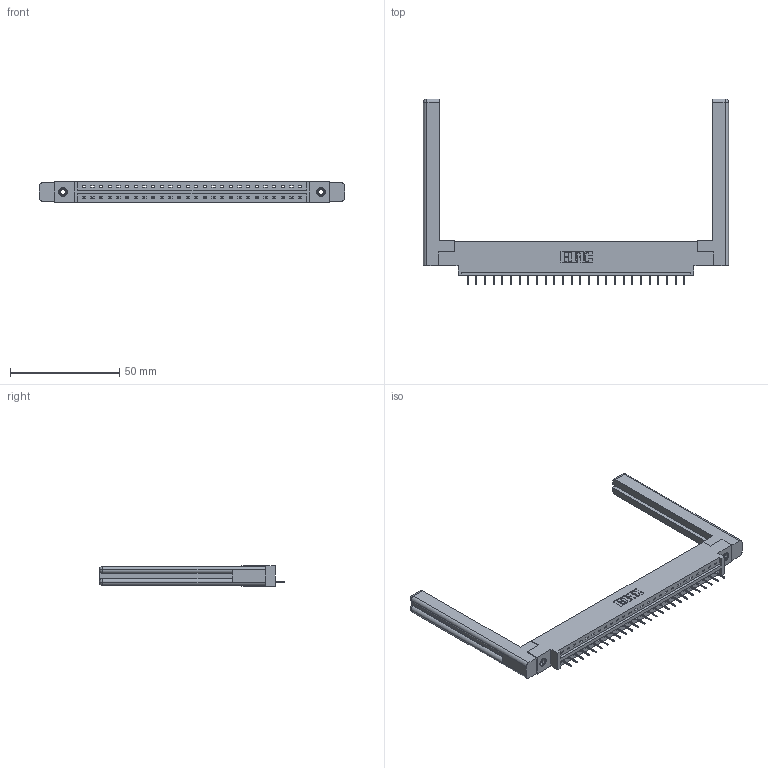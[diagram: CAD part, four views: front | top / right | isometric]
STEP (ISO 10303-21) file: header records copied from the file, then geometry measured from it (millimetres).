
FILE_DESCRIPTION (( 'STEP AP203' ), '1' );
FILE_NAME ('387-026-524-658.STEP', '2019-10-03T12:39:09', ( '' ), ( '' ), 'SwSTEP 2.0', 'SolidWorks 2016', '' );
FILE_SCHEMA (( 'CONFIG_CONTROL_DESIGN' ));
Length unit declared in the file: inch
Products named in the file (5): 345-250-001_345-250-001-102; 345-292-001_345-293-124; 337 Part_0.170 Offset - 0.156 Dia-TI; 307-220-058; 387-026-524-658
Assembly tree (31 placements, depth 2):
  387-026-524-658
    337 Part_0.170 Offset - 0.156 Dia-TI
    345-292-001_345-293-124  x26
    345-250-001_345-250-001-102  x2
    307-220-058  x2
Bounding box: 139.65 x 85.1 x 9.4 mm (x, y, z)
Volume: 21255.9 mm3; surface area: 19423.3 mm2
Topology: 31 solids, 31 shells, 1976 faces, 5669 edges, 3662 vertices
Faces by surface type: plane 1510, cylinder 442, cone 12, torus 12
Entity records: 24236 total; most frequent: CARTESIAN_POINT 4219, ORIENTED_EDGE 4120, DIRECTION 3604, EDGE_CURVE 2060, LINE 1888, VECTOR 1888, VERTEX_POINT 1362, AXIS2_PLACEMENT_3D 858
